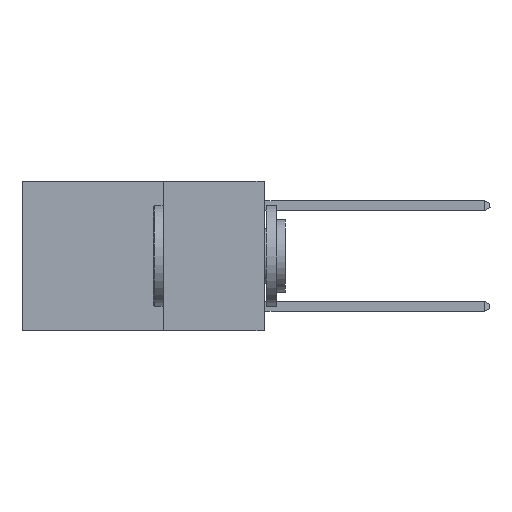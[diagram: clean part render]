
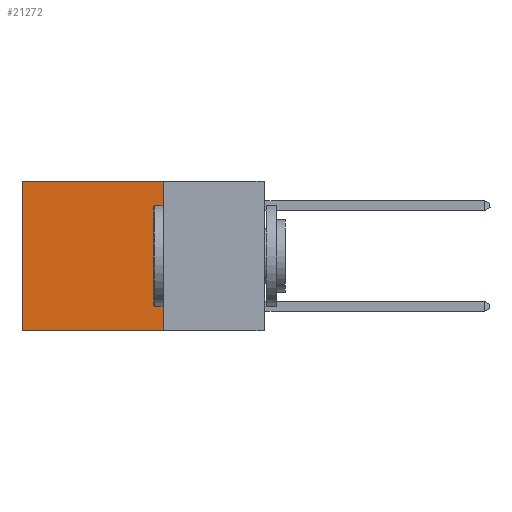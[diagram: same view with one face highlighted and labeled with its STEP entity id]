
A CAD part, left-side view. The second image highlights one B-rep face of the part: STEP entity #21272.
In plain terms, the highlighted planar face has unit normal (-1, 0, 0).
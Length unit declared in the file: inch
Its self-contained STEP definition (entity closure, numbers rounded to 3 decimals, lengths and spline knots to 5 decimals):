
#793 = CARTESIAN_POINT ( 'NONE',  ( 0.2625, 0.25, 0. ) ) ;
#2160 = VERTEX_POINT ( 'NONE', #25827 ) ;
#2683 = PLANE ( 'NONE',  #8664 ) ;
#3339 = EDGE_CURVE ( 'NONE', #25645, #19366, #19569, .T. ) ;
#3865 = CARTESIAN_POINT ( 'NONE',  ( 0.2625, 0.6, -0.37 ) ) ;
#3907 = ORIENTED_EDGE ( 'NONE', *, *, #3339, .F. ) ;
#4779 = LINE ( 'NONE', #10848, #18591 ) ;
#4844 = DIRECTION ( 'NONE',  ( 0., 0., -1. ) ) ;
#7226 = VECTOR ( 'NONE', #9911, 39.37008 ) ;
#8664 = AXIS2_PLACEMENT_3D ( 'NONE', #793, #17041, #4844 ) ;
#8666 = VECTOR ( 'NONE', #25261, 39.37008 ) ;
#9108 = ORIENTED_EDGE ( 'NONE', *, *, #13340, .T. ) ;
#9794 = DIRECTION ( 'NONE',  ( 0., 0., -1. ) ) ;
#9911 = DIRECTION ( 'NONE',  ( 0., 1., 0. ) ) ;
#10848 = CARTESIAN_POINT ( 'NONE',  ( 0.2625, 0.25, 0. ) ) ;
#11439 = CARTESIAN_POINT ( 'NONE',  ( 0.2625, 0.25, 0. ) ) ;
#12129 = CARTESIAN_POINT ( 'NONE',  ( 0.2625, 0.6, 0. ) ) ;
#13198 = CARTESIAN_POINT ( 'NONE',  ( 0.2625, 0.25, -0.37 ) ) ;
#13301 = ORIENTED_EDGE ( 'NONE', *, *, #22352, .F. ) ;
#13340 = EDGE_CURVE ( 'NONE', #25645, #2160, #4779, .T. ) ;
#13678 = CARTESIAN_POINT ( 'NONE',  ( 0.2625, 0.25, -0.37 ) ) ;
#14680 = FACE_OUTER_BOUND ( 'NONE', #19109, .T. ) ;
#14751 = CARTESIAN_POINT ( 'NONE',  ( 0.2625, 0.25, 0. ) ) ;
#15009 = VERTEX_POINT ( 'NONE', #3865 ) ;
#15581 = VECTOR ( 'NONE', #9794, 39.37008 ) ;
#16230 = LINE ( 'NONE', #13678, #7226 ) ;
#16871 = LINE ( 'NONE', #12129, #15581 ) ;
#16881 = DIRECTION ( 'NONE',  ( 0., 1., 0. ) ) ;
#17041 = DIRECTION ( 'NONE',  ( 1., 0., 0. ) ) ;
#18591 = VECTOR ( 'NONE', #16881, 39.37008 ) ;
#19109 = EDGE_LOOP ( 'NONE', ( #21908, #13301, #3907, #9108 ) ) ;
#19366 = VERTEX_POINT ( 'NONE', #13198 ) ;
#19569 = LINE ( 'NONE', #14751, #8666 ) ;
#21272 = ADVANCED_FACE ( 'NONE', ( #14680 ), #2683, .F. ) ;
#21667 = EDGE_CURVE ( 'NONE', #2160, #15009, #16871, .T. ) ;
#21908 = ORIENTED_EDGE ( 'NONE', *, *, #21667, .T. ) ;
#22352 = EDGE_CURVE ( 'NONE', #19366, #15009, #16230, .T. ) ;
#25261 = DIRECTION ( 'NONE',  ( 0., 0., -1. ) ) ;
#25645 = VERTEX_POINT ( 'NONE', #11439 ) ;
#25827 = CARTESIAN_POINT ( 'NONE',  ( 0.2625, 0.6, 0. ) ) ;
